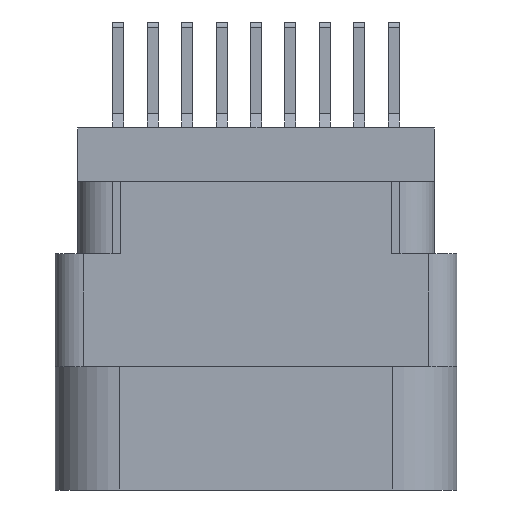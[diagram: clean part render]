
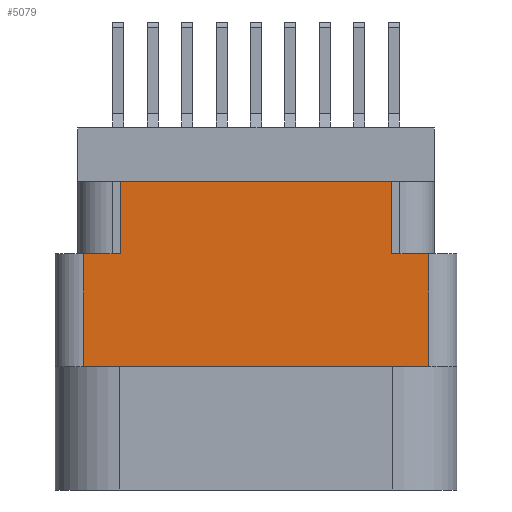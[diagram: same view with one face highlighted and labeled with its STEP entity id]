
A CAD part, left-side view. The second image highlights one B-rep face of the part: STEP entity #5079.
In plain terms, the highlighted planar face has unit normal (-1, 0, 0).
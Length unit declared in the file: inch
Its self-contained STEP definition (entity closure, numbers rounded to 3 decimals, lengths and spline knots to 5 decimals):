
#1677 = VECTOR ( 'NONE', #38868, 39.37008 ) ;
#2125 = CARTESIAN_POINT ( 'NONE',  ( -1.2955, -0.376, -0.274 ) ) ;
#3986 = EDGE_CURVE ( 'NONE', #30677, #4387, #34962, .T. ) ;
#4387 = VERTEX_POINT ( 'NONE', #2125 ) ;
#4908 = EDGE_CURVE ( 'NONE', #18369, #23502, #19401, .T. ) ;
#5079 = ADVANCED_FACE ( 'NONE', ( #8938 ), #15188, .T. ) ;
#5854 = EDGE_CURVE ( 'NONE', #30677, #26933, #17598, .T. ) ;
#7126 = CARTESIAN_POINT ( 'NONE',  ( -1.2955, 0., -0.274 ) ) ;
#7693 = CARTESIAN_POINT ( 'NONE',  ( -1.2955, 0.296, -0.274 ) ) ;
#8774 = ORIENTED_EDGE ( 'NONE', *, *, #16241, .F. ) ;
#8938 = FACE_OUTER_BOUND ( 'NONE', #37931, .T. ) ;
#9767 = DIRECTION ( 'NONE',  ( 0., 0., 1. ) ) ;
#10150 = CARTESIAN_POINT ( 'NONE',  ( -1.2955, -0.376, -0.52 ) ) ;
#11144 = VECTOR ( 'NONE', #17235, 39.37008 ) ;
#11651 = CARTESIAN_POINT ( 'NONE',  ( -1.2955, 0.376, -0.789 ) ) ;
#12801 = CARTESIAN_POINT ( 'NONE',  ( -1.2955, -0.376, -0.789 ) ) ;
#13645 = VECTOR ( 'NONE', #26976, 39.37008 ) ;
#14379 = VECTOR ( 'NONE', #9767, 39.37008 ) ;
#14698 = VERTEX_POINT ( 'NONE', #39026 ) ;
#15188 = PLANE ( 'NONE',  #27602 ) ;
#15498 = CARTESIAN_POINT ( 'NONE',  ( -1.2955, -0.296, -0.274 ) ) ;
#16081 = CARTESIAN_POINT ( 'NONE',  ( -1.2955, 0., -0.274 ) ) ;
#16241 = EDGE_CURVE ( 'NONE', #41581, #4387, #39720, .T. ) ;
#16384 = CARTESIAN_POINT ( 'NONE',  ( -1.2955, 0.376, -0.274 ) ) ;
#16496 = VECTOR ( 'NONE', #19498, 39.37008 ) ;
#17235 = DIRECTION ( 'NONE',  ( 0., -1., 0. ) ) ;
#17598 = LINE ( 'NONE', #34761, #1677 ) ;
#18369 = VERTEX_POINT ( 'NONE', #16384 ) ;
#18763 = DIRECTION ( 'NONE',  ( 0., 0., 1. ) ) ;
#18946 = CARTESIAN_POINT ( 'NONE',  ( -1.2955, -0.296, -0.117 ) ) ;
#19401 = LINE ( 'NONE', #7126, #11144 ) ;
#19498 = DIRECTION ( 'NONE',  ( 0., 0., 1. ) ) ;
#20284 = LINE ( 'NONE', #23401, #13645 ) ;
#20368 = ORIENTED_EDGE ( 'NONE', *, *, #42375, .F. ) ;
#22295 = DIRECTION ( 'NONE',  ( -1., 0., 0. ) ) ;
#23401 = CARTESIAN_POINT ( 'NONE',  ( -1.2955, 0.438, -0.117 ) ) ;
#23502 = VERTEX_POINT ( 'NONE', #7693 ) ;
#24175 = CARTESIAN_POINT ( 'NONE',  ( -1.2955, -0.296, -0.274 ) ) ;
#25577 = ORIENTED_EDGE ( 'NONE', *, *, #25845, .T. ) ;
#25837 = CARTESIAN_POINT ( 'NONE',  ( -1.2955, -0.438, -0.789 ) ) ;
#25845 = EDGE_CURVE ( 'NONE', #41581, #33222, #43559, .T. ) ;
#26911 = CARTESIAN_POINT ( 'NONE',  ( -1.2955, 0.376, -0.52 ) ) ;
#26933 = VERTEX_POINT ( 'NONE', #26911 ) ;
#26976 = DIRECTION ( 'NONE',  ( 0., -1., 0. ) ) ;
#27602 = AXIS2_PLACEMENT_3D ( 'NONE', #25837, #22295, #18763 ) ;
#29135 = ORIENTED_EDGE ( 'NONE', *, *, #4908, .F. ) ;
#29561 = EDGE_CURVE ( 'NONE', #18369, #26933, #44159, .T. ) ;
#29981 = DIRECTION ( 'NONE',  ( 0., 0., -1. ) ) ;
#29983 = DIRECTION ( 'NONE',  ( 0., -1., 0. ) ) ;
#30677 = VERTEX_POINT ( 'NONE', #10150 ) ;
#31190 = EDGE_CURVE ( 'NONE', #23502, #14698, #31433, .T. ) ;
#31433 = LINE ( 'NONE', #43784, #16496 ) ;
#32654 = ORIENTED_EDGE ( 'NONE', *, *, #31190, .F. ) ;
#33222 = VERTEX_POINT ( 'NONE', #18946 ) ;
#34761 = CARTESIAN_POINT ( 'NONE',  ( -1.2955, 0., -0.52 ) ) ;
#34824 = ORIENTED_EDGE ( 'NONE', *, *, #29561, .T. ) ;
#34962 = LINE ( 'NONE', #12801, #41509 ) ;
#35415 = ORIENTED_EDGE ( 'NONE', *, *, #5854, .F. ) ;
#37413 = DIRECTION ( 'NONE',  ( 0., 0., 1. ) ) ;
#37931 = EDGE_LOOP ( 'NONE', ( #29135, #34824, #35415, #42227, #8774, #25577, #20368, #32654 ) ) ;
#38868 = DIRECTION ( 'NONE',  ( 0., 1., 0. ) ) ;
#39026 = CARTESIAN_POINT ( 'NONE',  ( -1.2955, 0.296, -0.117 ) ) ;
#39720 = LINE ( 'NONE', #16081, #41899 ) ;
#39807 = VECTOR ( 'NONE', #29981, 39.37008 ) ;
#41509 = VECTOR ( 'NONE', #37413, 39.37008 ) ;
#41581 = VERTEX_POINT ( 'NONE', #24175 ) ;
#41899 = VECTOR ( 'NONE', #29983, 39.37008 ) ;
#42227 = ORIENTED_EDGE ( 'NONE', *, *, #3986, .T. ) ;
#42375 = EDGE_CURVE ( 'NONE', #14698, #33222, #20284, .T. ) ;
#43559 = LINE ( 'NONE', #15498, #14379 ) ;
#43784 = CARTESIAN_POINT ( 'NONE',  ( -1.2955, 0.296, -0.274 ) ) ;
#44159 = LINE ( 'NONE', #11651, #39807 ) ;
